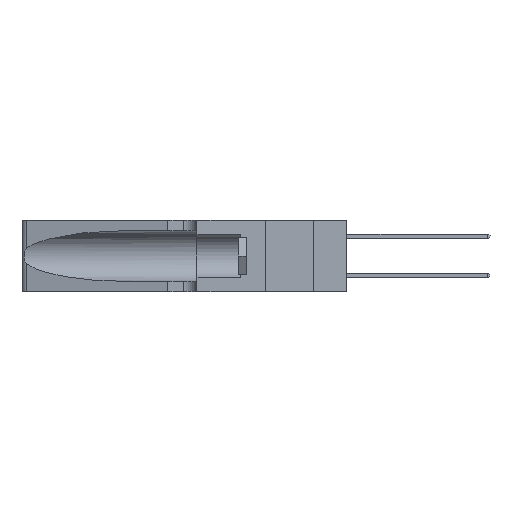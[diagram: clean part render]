
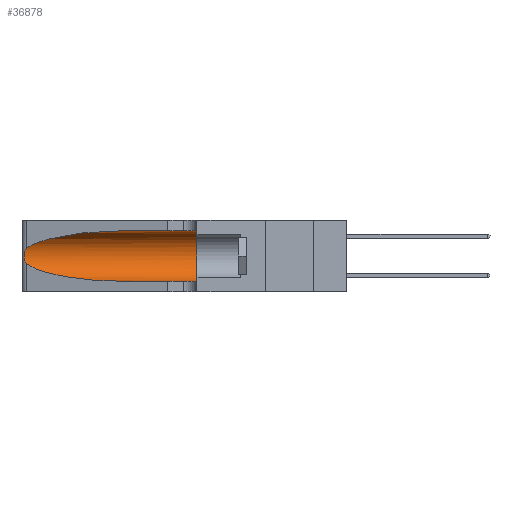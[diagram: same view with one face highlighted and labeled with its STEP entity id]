
A CAD part, left-side view. The second image highlights one B-rep face of the part: STEP entity #36878.
In plain terms, the highlighted cylindrical face has radius 3.308 mm (diameter 6.617 mm), a partial arc.
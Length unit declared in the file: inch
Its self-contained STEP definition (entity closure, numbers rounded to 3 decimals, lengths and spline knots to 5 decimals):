
#60 = EDGE_LOOP ( 'NONE', ( #1900, #20964, #26908, #35260, #15705, #29805 ) ) ;
#91 = CARTESIAN_POINT ( 'NONE',  ( 0.1305, 0.35, 0.185 ) ) ;
#1009 = CYLINDRICAL_SURFACE ( 'NONE', #27764, 0.13025 ) ;
#1900 = ORIENTED_EDGE ( 'NONE', *, *, #18256, .T. ) ;
#1974 = FACE_OUTER_BOUND ( 'NONE', #60, .T. ) ;
#2670 = CARTESIAN_POINT ( 'NONE',  ( 0.25789, 1.23486, 0.15765 ) ) ;
#3845 = CARTESIAN_POINT ( 'NONE',  ( 0.25487, 1.22718, 0.14631 ) ) ;
#3846 = CARTESIAN_POINT ( 'NONE',  ( 0.25555, 1.22994, 0.2215 ) ) ;
#4584 = CARTESIAN_POINT ( 'NONE',  ( 0.1305, 1.61858, 0.05475 ) ) ;
#4725 = CARTESIAN_POINT ( 'NONE',  ( 0.25787, 1.23484, 0.2124 ) ) ;
#5422 = VERTEX_POINT ( 'NONE', #25843 ) ;
#6238 = DIRECTION ( 'NONE',  ( 0., -1., 0. ) ) ;
#7619 = CARTESIAN_POINT ( 'NONE',  ( 0.25854, 1.2359, 0.20912 ) ) ;
#7676 = CARTESIAN_POINT ( 'NONE',  ( 0.1305, 0.35, 0.05475 ) ) ;
#8918 = CARTESIAN_POINT ( 'NONE',  ( 0.25487, 1.22718, 0.22369 ) ) ;
#10651 = B_SPLINE_CURVE_WITH_KNOTS ( 'NONE', 3,
 ( #27575, #3846, #16416, #4725, #7619, #16537, #28206, #14099, #31277, #11290, #2670, #16789, #26642, #18149 ),
 .UNSPECIFIED., .F., .F.,
 ( 4, 2, 2, 2, 2, 2, 4 ),
 ( 0., 0.00027, 0.00053, 0.00107, 0.0016, 0.00187, 0.00214 ),
 .UNSPECIFIED. ) ;
#11290 = CARTESIAN_POINT ( 'NONE',  ( 0.25856, 1.23593, 0.16098 ) ) ;
#11681 = VECTOR ( 'NONE', #33953, 39.37008 ) ;
#11734 = LINE ( 'NONE', #18828, #34961 ) ;
#12143 = EDGE_CURVE ( 'NONE', #5422, #27527, #11734, .T. ) ;
#12411 = VERTEX_POINT ( 'NONE', #3845 ) ;
#12514 = CARTESIAN_POINT ( 'NONE',  ( 0.2373, 1.15595, 0.28018 ) ) ;
#14099 = CARTESIAN_POINT ( 'NONE',  ( 0.26075, 1.23896, 0.178 ) ) ;
#14106 = CARTESIAN_POINT ( 'NONE',  ( 0.2373, 1.15595, 0.08982 ) ) ;
#15602 = CARTESIAN_POINT ( 'NONE',  ( 0.25487, 1.22718, 0.22369 ) ) ;
#15705 = ORIENTED_EDGE ( 'NONE', *, *, #27628, .F. ) ;
#16416 = CARTESIAN_POINT ( 'NONE',  ( 0.25639, 1.23184, 0.21858 ) ) ;
#16537 = CARTESIAN_POINT ( 'NONE',  ( 0.26018, 1.23835, 0.19895 ) ) ;
#16789 = CARTESIAN_POINT ( 'NONE',  ( 0.25639, 1.23186, 0.15144 ) ) ;
#17964 = CARTESIAN_POINT ( 'NONE',  ( 0.1305, 1.61858, 0.185 ) ) ;
#18149 = CARTESIAN_POINT ( 'NONE',  ( 0.25487, 1.22718, 0.14631 ) ) ;
#18211 = CARTESIAN_POINT ( 'NONE',  ( 0.1305, 0.72297, 0.05475 ) ) ;
#18256 = EDGE_CURVE ( 'NONE', #5422, #36697, #26959, .T. ) ;
#18828 = CARTESIAN_POINT ( 'NONE',  ( 0.1305, 1.61858, 0.31525 ) ) ;
#19473 = VERTEX_POINT ( 'NONE', #7676 ) ;
#20964 = ORIENTED_EDGE ( 'NONE', *, *, #24198, .T. ) ;
#20995 = CIRCLE ( 'NONE', #27609, 0.13025 ) ;
#21209 = CARTESIAN_POINT ( 'NONE',  ( 0.1305, 0.72297, 0.31525 ) ) ;
#21270 = LINE ( 'NONE', #4584, #11681 ) ;
#21889 =( BOUNDED_CURVE ( )  B_SPLINE_CURVE ( 3, ( #34735, #14106, #28873, #28754 ),
 .UNSPECIFIED., .F., .F. ) 
 B_SPLINE_CURVE_WITH_KNOTS ( ( 4, 4 ),
 ( 3.44316, 4.71239 ),
 .UNSPECIFIED. ) 
 CURVE ( )  GEOMETRIC_REPRESENTATION_ITEM ( )  RATIONAL_B_SPLINE_CURVE ( ( 1., 0.87, 0.87, 1. ) ) 
 REPRESENTATION_ITEM ( '' )  );
#24198 = EDGE_CURVE ( 'NONE', #36697, #12411, #10651, .T. ) ;
#24647 = EDGE_CURVE ( 'NONE', #36910, #19473, #21270, .T. ) ;
#25835 = EDGE_CURVE ( 'NONE', #12411, #36910, #21889, .T. ) ;
#25843 = CARTESIAN_POINT ( 'NONE',  ( 0.1305, 0.72297, 0.31525 ) ) ;
#26514 = CARTESIAN_POINT ( 'NONE',  ( 0.18966, 0.96281, 0.31525 ) ) ;
#26580 = DIRECTION ( 'NONE',  ( 0., 0., -1. ) ) ;
#26642 = CARTESIAN_POINT ( 'NONE',  ( 0.25555, 1.22993, 0.14849 ) ) ;
#26908 = ORIENTED_EDGE ( 'NONE', *, *, #25835, .T. ) ;
#26959 =( BOUNDED_CURVE ( )  B_SPLINE_CURVE ( 3, ( #21209, #26514, #12514, #15602 ),
 .UNSPECIFIED., .F., .F. ) 
 B_SPLINE_CURVE_WITH_KNOTS ( ( 4, 4 ),
 ( 1.5708, 2.84003 ),
 .UNSPECIFIED. ) 
 CURVE ( )  GEOMETRIC_REPRESENTATION_ITEM ( )  RATIONAL_B_SPLINE_CURVE ( ( 1., 0.87, 0.87, 1. ) ) 
 REPRESENTATION_ITEM ( '' )  );
#27527 = VERTEX_POINT ( 'NONE', #31673 ) ;
#27575 = CARTESIAN_POINT ( 'NONE',  ( 0.25487, 1.22718, 0.22369 ) ) ;
#27609 = AXIS2_PLACEMENT_3D ( 'NONE', #91, #34970, #32028 ) ;
#27628 = EDGE_CURVE ( 'NONE', #27527, #19473, #20995, .T. ) ;
#27764 = AXIS2_PLACEMENT_3D ( 'NONE', #17964, #6238, #26580 ) ;
#28206 = CARTESIAN_POINT ( 'NONE',  ( 0.26075, 1.23896, 0.19203 ) ) ;
#28348 = DIRECTION ( 'NONE',  ( 0., -1., 0. ) ) ;
#28754 = CARTESIAN_POINT ( 'NONE',  ( 0.1305, 0.72297, 0.05475 ) ) ;
#28873 = CARTESIAN_POINT ( 'NONE',  ( 0.18966, 0.96281, 0.05475 ) ) ;
#29805 = ORIENTED_EDGE ( 'NONE', *, *, #12143, .F. ) ;
#31277 = CARTESIAN_POINT ( 'NONE',  ( 0.26017, 1.23833, 0.17102 ) ) ;
#31673 = CARTESIAN_POINT ( 'NONE',  ( 0.1305, 0.35, 0.31525 ) ) ;
#32028 = DIRECTION ( 'NONE',  ( 0., 0., 1. ) ) ;
#33953 = DIRECTION ( 'NONE',  ( 0., -1., 0. ) ) ;
#34735 = CARTESIAN_POINT ( 'NONE',  ( 0.25487, 1.22718, 0.14631 ) ) ;
#34961 = VECTOR ( 'NONE', #28348, 39.37008 ) ;
#34970 = DIRECTION ( 'NONE',  ( 0., 1., 0. ) ) ;
#35260 = ORIENTED_EDGE ( 'NONE', *, *, #24647, .T. ) ;
#36697 = VERTEX_POINT ( 'NONE', #8918 ) ;
#36878 = ADVANCED_FACE ( 'NONE', ( #1974 ), #1009, .F. ) ;
#36910 = VERTEX_POINT ( 'NONE', #18211 ) ;
